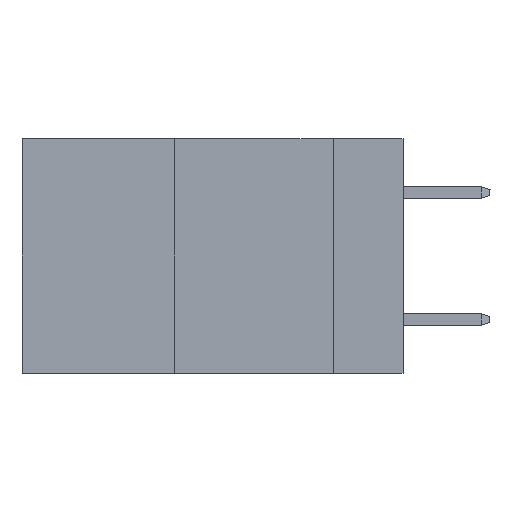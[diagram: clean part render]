
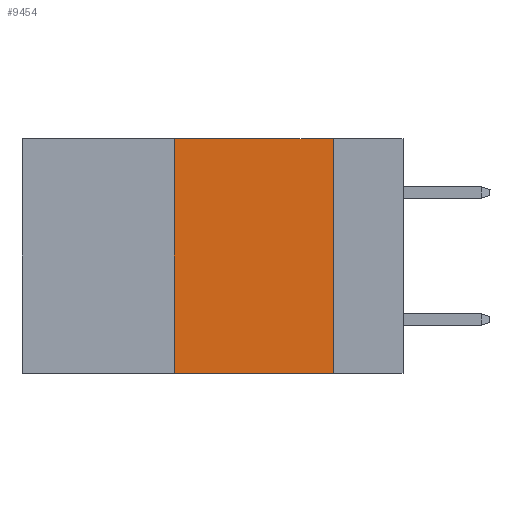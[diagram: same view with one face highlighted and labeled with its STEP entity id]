
A CAD part, left-side view. The second image highlights one B-rep face of the part: STEP entity #9454.
In plain terms, the highlighted planar face has unit normal (-1, 0, 0).
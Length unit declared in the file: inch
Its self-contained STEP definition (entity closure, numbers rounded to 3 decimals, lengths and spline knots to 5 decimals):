
#77 = CARTESIAN_POINT ( 'NONE',  ( 0., 0.36, 0. ) ) ;
#698 = LINE ( 'NONE', #9733, #10176 ) ;
#1352 = CARTESIAN_POINT ( 'NONE',  ( 0., 0.6, 0. ) ) ;
#1422 = VERTEX_POINT ( 'NONE', #8299 ) ;
#1470 = VECTOR ( 'NONE', #4096, 39.37008 ) ;
#1790 = VECTOR ( 'NONE', #6885, 39.37008 ) ;
#1838 = VERTEX_POINT ( 'NONE', #5246 ) ;
#1927 = ORIENTED_EDGE ( 'NONE', *, *, #11495, .F. ) ;
#2222 = CARTESIAN_POINT ( 'NONE',  ( 0., 0.6, -0.37 ) ) ;
#2242 = FACE_OUTER_BOUND ( 'NONE', #8381, .T. ) ;
#2375 = ORIENTED_EDGE ( 'NONE', *, *, #11696, .T. ) ;
#2443 = LINE ( 'NONE', #2222, #1470 ) ;
#2545 = EDGE_CURVE ( 'NONE', #2899, #1422, #5750, .T. ) ;
#2899 = VERTEX_POINT ( 'NONE', #11364 ) ;
#3666 = DIRECTION ( 'NONE',  ( 0., 0., 1. ) ) ;
#3987 = CARTESIAN_POINT ( 'NONE',  ( 0., 0.36, -0.37 ) ) ;
#4096 = DIRECTION ( 'NONE',  ( 0., -1., 0. ) ) ;
#5246 = CARTESIAN_POINT ( 'NONE',  ( 0., 0.36, 0. ) ) ;
#5750 = LINE ( 'NONE', #11275, #1790 ) ;
#5856 = DIRECTION ( 'NONE',  ( 0., 0., -1. ) ) ;
#6885 = DIRECTION ( 'NONE',  ( 0., 0., -1. ) ) ;
#7344 = EDGE_CURVE ( 'NONE', #1838, #2899, #698, .T. ) ;
#7642 = PLANE ( 'NONE',  #9242 ) ;
#8299 = CARTESIAN_POINT ( 'NONE',  ( 0., 0.11, -0.37 ) ) ;
#8381 = EDGE_LOOP ( 'NONE', ( #8724, #9303, #1927, #2375 ) ) ;
#8724 = ORIENTED_EDGE ( 'NONE', *, *, #2545, .F. ) ;
#9102 = LINE ( 'NONE', #77, #10369 ) ;
#9242 = AXIS2_PLACEMENT_3D ( 'NONE', #1352, #9301, #5856 ) ;
#9301 = DIRECTION ( 'NONE',  ( 1., 0., 0. ) ) ;
#9303 = ORIENTED_EDGE ( 'NONE', *, *, #7344, .F. ) ;
#9454 = ADVANCED_FACE ( 'NONE', ( #2242 ), #7642, .F. ) ;
#9733 = CARTESIAN_POINT ( 'NONE',  ( 0., 0.6, 0. ) ) ;
#9762 = VERTEX_POINT ( 'NONE', #3987 ) ;
#10176 = VECTOR ( 'NONE', #11567, 39.37008 ) ;
#10369 = VECTOR ( 'NONE', #3666, 39.37008 ) ;
#11275 = CARTESIAN_POINT ( 'NONE',  ( 0., 0.11, 0. ) ) ;
#11364 = CARTESIAN_POINT ( 'NONE',  ( 0., 0.11, 0. ) ) ;
#11495 = EDGE_CURVE ( 'NONE', #9762, #1838, #9102, .T. ) ;
#11567 = DIRECTION ( 'NONE',  ( 0., -1., 0. ) ) ;
#11696 = EDGE_CURVE ( 'NONE', #9762, #1422, #2443, .T. ) ;
